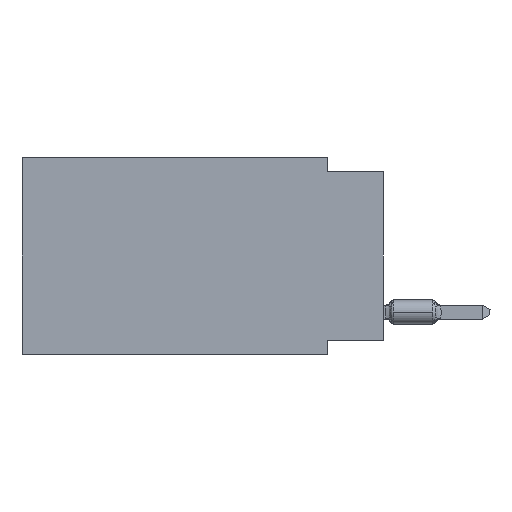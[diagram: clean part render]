
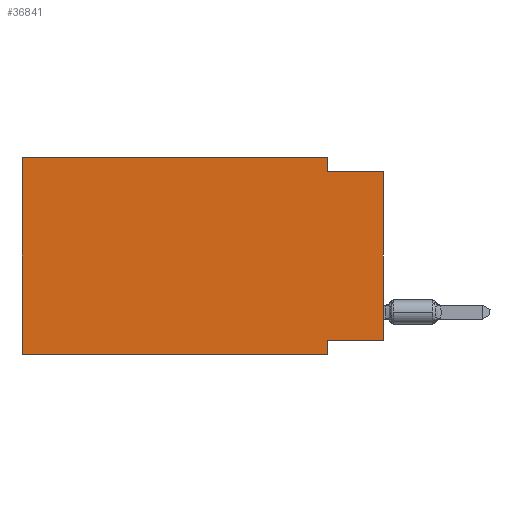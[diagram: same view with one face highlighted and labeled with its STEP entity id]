
A CAD part, left-side view. The second image highlights one B-rep face of the part: STEP entity #36841.
In plain terms, the highlighted planar face has unit normal (-1, 0, 0).
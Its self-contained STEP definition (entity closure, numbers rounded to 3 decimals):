
#139 = EDGE_CURVE ( 'NONE', #3292, #23097, #3431, .T. ) ;
#600 = ORIENTED_EDGE ( 'NONE', *, *, #21700, .F. ) ;
#718 = CARTESIAN_POINT ( 'NONE',  ( 0., 2.54, 0. ) ) ;
#1359 = CARTESIAN_POINT ( 'NONE',  ( 0., 2.54, -8.255 ) ) ;
#1423 = LINE ( 'NONE', #21039, #20816 ) ;
#1994 = EDGE_CURVE ( 'NONE', #3292, #26519, #3417, .T. ) ;
#2910 = DIRECTION ( 'NONE',  ( 0., 0., 1. ) ) ;
#3292 = VERTEX_POINT ( 'NONE', #39092 ) ;
#3417 = LINE ( 'NONE', #6910, #7028 ) ;
#3431 = LINE ( 'NONE', #44875, #31479 ) ;
#3464 = CARTESIAN_POINT ( 'NONE',  ( 0., 16.383, -8.89 ) ) ;
#3624 = DIRECTION ( 'NONE',  ( 0., -1., 0. ) ) ;
#3746 = CARTESIAN_POINT ( 'NONE',  ( 0., 2.54, -8.89 ) ) ;
#3992 = VERTEX_POINT ( 'NONE', #24585 ) ;
#4071 = VERTEX_POINT ( 'NONE', #3464 ) ;
#6910 = CARTESIAN_POINT ( 'NONE',  ( 0., 0., 0. ) ) ;
#7028 = VECTOR ( 'NONE', #21827, 1000. ) ;
#7137 = VECTOR ( 'NONE', #35025, 1000. ) ;
#7747 = VERTEX_POINT ( 'NONE', #3746 ) ;
#10022 = DIRECTION ( 'NONE',  ( 0., -1., 0. ) ) ;
#10105 = CARTESIAN_POINT ( 'NONE',  ( 0., 16.383, 0. ) ) ;
#10485 = AXIS2_PLACEMENT_3D ( 'NONE', #35377, #12552, #32399 ) ;
#10737 = VECTOR ( 'NONE', #2910, 1000. ) ;
#10739 = EDGE_CURVE ( 'NONE', #4071, #3992, #45050, .T. ) ;
#11317 = CARTESIAN_POINT ( 'NONE',  ( 0., 16.383, 0. ) ) ;
#12453 = EDGE_CURVE ( 'NONE', #23097, #7747, #12713, .T. ) ;
#12552 = DIRECTION ( 'NONE',  ( 1., 0., 0. ) ) ;
#12713 = LINE ( 'NONE', #27612, #7137 ) ;
#13188 = VECTOR ( 'NONE', #10022, 1000. ) ;
#14262 = ORIENTED_EDGE ( 'NONE', *, *, #12453, .F. ) ;
#15303 = ORIENTED_EDGE ( 'NONE', *, *, #10739, .F. ) ;
#15542 = EDGE_CURVE ( 'NONE', #4071, #7747, #1423, .T. ) ;
#16251 = ORIENTED_EDGE ( 'NONE', *, *, #1994, .T. ) ;
#17011 = PLANE ( 'NONE',  #10485 ) ;
#17582 = EDGE_CURVE ( 'NONE', #34797, #25489, #40899, .T. ) ;
#20816 = VECTOR ( 'NONE', #32201, 1000. ) ;
#21039 = CARTESIAN_POINT ( 'NONE',  ( 0., 16.383, -8.89 ) ) ;
#21700 = EDGE_CURVE ( 'NONE', #3992, #34797, #48282, .T. ) ;
#21827 = DIRECTION ( 'NONE',  ( 0., 0., 1. ) ) ;
#22065 = CARTESIAN_POINT ( 'NONE',  ( 0., 2.54, 0. ) ) ;
#22391 = EDGE_LOOP ( 'NONE', ( #16251, #45184, #41248, #600, #15303, #23380, #14262, #29132 ) ) ;
#23097 = VERTEX_POINT ( 'NONE', #1359 ) ;
#23380 = ORIENTED_EDGE ( 'NONE', *, *, #15542, .T. ) ;
#24585 = CARTESIAN_POINT ( 'NONE',  ( 0., 16.383, 0. ) ) ;
#24714 = FACE_OUTER_BOUND ( 'NONE', #22391, .T. ) ;
#25489 = VERTEX_POINT ( 'NONE', #38471 ) ;
#26519 = VERTEX_POINT ( 'NONE', #47527 ) ;
#27612 = CARTESIAN_POINT ( 'NONE',  ( 0., 2.54, -8.89 ) ) ;
#28876 = LINE ( 'NONE', #43994, #13188 ) ;
#29132 = ORIENTED_EDGE ( 'NONE', *, *, #139, .F. ) ;
#31479 = VECTOR ( 'NONE', #33460, 1000. ) ;
#32201 = DIRECTION ( 'NONE',  ( 0., -1., 0. ) ) ;
#32399 = DIRECTION ( 'NONE',  ( 0., 0., -1. ) ) ;
#33460 = DIRECTION ( 'NONE',  ( 0., 1., 0. ) ) ;
#34797 = VERTEX_POINT ( 'NONE', #718 ) ;
#35025 = DIRECTION ( 'NONE',  ( 0., 0., -1. ) ) ;
#35090 = VECTOR ( 'NONE', #37156, 1000. ) ;
#35377 = CARTESIAN_POINT ( 'NONE',  ( 0., 16.383, 0. ) ) ;
#36841 = ADVANCED_FACE ( 'NONE', ( #24714 ), #17011, .F. ) ;
#37156 = DIRECTION ( 'NONE',  ( 0., 0., -1. ) ) ;
#38471 = CARTESIAN_POINT ( 'NONE',  ( 0., 2.54, -0.635 ) ) ;
#38689 = EDGE_CURVE ( 'NONE', #25489, #26519, #28876, .T. ) ;
#39092 = CARTESIAN_POINT ( 'NONE',  ( 0., 0., -8.255 ) ) ;
#40899 = LINE ( 'NONE', #22065, #35090 ) ;
#41248 = ORIENTED_EDGE ( 'NONE', *, *, #17582, .F. ) ;
#43994 = CARTESIAN_POINT ( 'NONE',  ( 0., 0., -0.635 ) ) ;
#44875 = CARTESIAN_POINT ( 'NONE',  ( 0., 0., -8.255 ) ) ;
#45050 = LINE ( 'NONE', #10105, #10737 ) ;
#45184 = ORIENTED_EDGE ( 'NONE', *, *, #38689, .F. ) ;
#47271 = VECTOR ( 'NONE', #3624, 1000. ) ;
#47527 = CARTESIAN_POINT ( 'NONE',  ( 0., 0., -0.635 ) ) ;
#48282 = LINE ( 'NONE', #11317, #47271 ) ;
